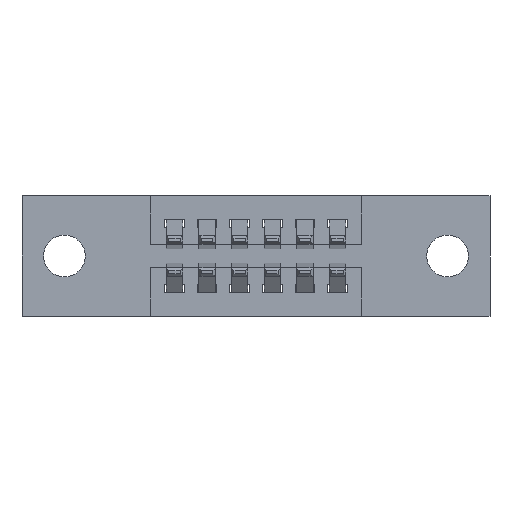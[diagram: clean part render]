
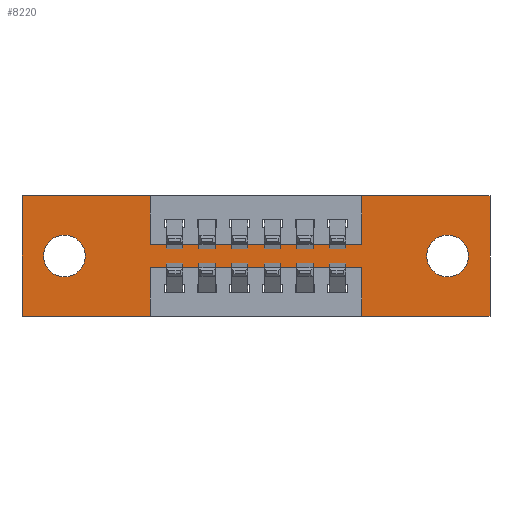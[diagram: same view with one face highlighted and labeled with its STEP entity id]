
A CAD part, front view. The second image highlights one B-rep face of the part: STEP entity #8220.
In plain terms, the highlighted planar face has unit normal (0, -1, 0).
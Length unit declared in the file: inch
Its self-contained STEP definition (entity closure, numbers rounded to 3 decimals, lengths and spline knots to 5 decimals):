
#97 = VERTEX_POINT ( 'NONE', #9076 ) ;
#116 = CARTESIAN_POINT ( 'NONE',  ( 1.305, 0., -0.249 ) ) ;
#131 = EDGE_CURVE ( 'NONE', #3369, #7412, #6602, .T. ) ;
#133 = LINE ( 'NONE', #6374, #9207 ) ;
#160 = CARTESIAN_POINT ( 'NONE',  ( 0.3925, 0., -0.22 ) ) ;
#163 = ORIENTED_EDGE ( 'NONE', *, *, #3945, .T. ) ;
#171 = DIRECTION ( 'NONE',  ( 0., 1., 0. ) ) ;
#182 = CARTESIAN_POINT ( 'NONE',  ( 0.3925, 0., -0.22 ) ) ;
#238 = CARTESIAN_POINT ( 'NONE',  ( 1.0425, 0., 0. ) ) ;
#259 = VECTOR ( 'NONE', #5340, 39.37008 ) ;
#364 = ORIENTED_EDGE ( 'NONE', *, *, #7373, .F. ) ;
#404 = DIRECTION ( 'NONE',  ( 0., 0., 1. ) ) ;
#483 = CARTESIAN_POINT ( 'NONE',  ( 0., 0., 0. ) ) ;
#496 = VERTEX_POINT ( 'NONE', #1741 ) ;
#575 = CARTESIAN_POINT ( 'NONE',  ( 1.305, 0., -0.185 ) ) ;
#585 = CARTESIAN_POINT ( 'NONE',  ( 0., 0., -0.37 ) ) ;
#763 = VECTOR ( 'NONE', #7663, 39.37008 ) ;
#859 = CIRCLE ( 'NONE', #6962, 0.064 ) ;
#992 = VERTEX_POINT ( 'NONE', #6722 ) ;
#1014 = VERTEX_POINT ( 'NONE', #182 ) ;
#1096 = CARTESIAN_POINT ( 'NONE',  ( 1.435, 0., 0. ) ) ;
#1185 = CARTESIAN_POINT ( 'NONE',  ( 1.0425, 0., -0.37 ) ) ;
#1200 = VERTEX_POINT ( 'NONE', #9214 ) ;
#1331 = VERTEX_POINT ( 'NONE', #1185 ) ;
#1410 = LINE ( 'NONE', #160, #9097 ) ;
#1441 = CARTESIAN_POINT ( 'NONE',  ( 0., 0., 0. ) ) ;
#1536 = CARTESIAN_POINT ( 'NONE',  ( 1.0425, 0., 0. ) ) ;
#1552 = EDGE_CURVE ( 'NONE', #97, #4890, #8085, .T. ) ;
#1741 = CARTESIAN_POINT ( 'NONE',  ( 1.0425, 0., -0.22 ) ) ;
#1841 = EDGE_LOOP ( 'NONE', ( #163, #6356 ) ) ;
#1906 = DIRECTION ( 'NONE',  ( 0., 0., -1. ) ) ;
#1920 = ORIENTED_EDGE ( 'NONE', *, *, #7056, .F. ) ;
#2049 = ORIENTED_EDGE ( 'NONE', *, *, #8981, .F. ) ;
#2123 = ORIENTED_EDGE ( 'NONE', *, *, #3942, .F. ) ;
#2144 = EDGE_CURVE ( 'NONE', #4339, #3369, #4245, .T. ) ;
#2242 = LINE ( 'NONE', #4698, #3986 ) ;
#2432 = EDGE_CURVE ( 'NONE', #7024, #2604, #133, .T. ) ;
#2460 = ORIENTED_EDGE ( 'NONE', *, *, #131, .F. ) ;
#2490 = EDGE_LOOP ( 'NONE', ( #2498, #3957, #364, #5927, #2123, #2460, #6778, #5373, #7607, #2049, #6780, #1920 ) ) ;
#2498 = ORIENTED_EDGE ( 'NONE', *, *, #2923, .F. ) ;
#2604 = VERTEX_POINT ( 'NONE', #5002 ) ;
#2683 = ORIENTED_EDGE ( 'NONE', *, *, #6058, .T. ) ;
#2715 = FACE_BOUND ( 'NONE', #1841, .T. ) ;
#2771 = EDGE_CURVE ( 'NONE', #496, #1014, #1410, .T. ) ;
#2819 = VECTOR ( 'NONE', #7422, 39.37008 ) ;
#2849 = LINE ( 'NONE', #1096, #4599 ) ;
#2923 = EDGE_CURVE ( 'NONE', #1014, #5334, #2242, .T. ) ;
#2934 = DIRECTION ( 'NONE',  ( 0., 1., 0. ) ) ;
#2957 = CIRCLE ( 'NONE', #9351, 0.064 ) ;
#3071 = EDGE_CURVE ( 'NONE', #992, #1331, #8165, .T. ) ;
#3369 = VERTEX_POINT ( 'NONE', #238 ) ;
#3648 = DIRECTION ( 'NONE',  ( 1., 0., 0. ) ) ;
#3942 = EDGE_CURVE ( 'NONE', #7412, #992, #2849, .T. ) ;
#3945 = EDGE_CURVE ( 'NONE', #8912, #9149, #2957, .T. ) ;
#3957 = ORIENTED_EDGE ( 'NONE', *, *, #2771, .F. ) ;
#3986 = VECTOR ( 'NONE', #5474, 39.37008 ) ;
#4027 = EDGE_LOOP ( 'NONE', ( #6821, #2683 ) ) ;
#4134 = PLANE ( 'NONE',  #7288 ) ;
#4175 = VERTEX_POINT ( 'NONE', #116 ) ;
#4245 = LINE ( 'NONE', #1536, #259 ) ;
#4307 = DIRECTION ( 'NONE',  ( -1., 0., 0. ) ) ;
#4339 = VERTEX_POINT ( 'NONE', #5133 ) ;
#4340 = AXIS2_PLACEMENT_3D ( 'NONE', #575, #2934, #7323 ) ;
#4599 = VECTOR ( 'NONE', #5661, 39.37008 ) ;
#4657 = DIRECTION ( 'NONE',  ( 0., 0., -1. ) ) ;
#4698 = CARTESIAN_POINT ( 'NONE',  ( 0.3925, 0., -0.37 ) ) ;
#4736 = CARTESIAN_POINT ( 'NONE',  ( 0., 0., 0. ) ) ;
#4763 = DIRECTION ( 'NONE',  ( 0., 0., 1. ) ) ;
#4890 = VERTEX_POINT ( 'NONE', #483 ) ;
#4946 = VECTOR ( 'NONE', #4959, 39.37008 ) ;
#4959 = DIRECTION ( 'NONE',  ( -1., 0., 0. ) ) ;
#5002 = CARTESIAN_POINT ( 'NONE',  ( 0.3925, 0., -0.15 ) ) ;
#5133 = CARTESIAN_POINT ( 'NONE',  ( 1.0425, 0., -0.15 ) ) ;
#5173 = LINE ( 'NONE', #585, #4946 ) ;
#5334 = VERTEX_POINT ( 'NONE', #8488 ) ;
#5340 = DIRECTION ( 'NONE',  ( 0., 0., 1. ) ) ;
#5373 = ORIENTED_EDGE ( 'NONE', *, *, #9313, .F. ) ;
#5474 = DIRECTION ( 'NONE',  ( 0., 0., -1. ) ) ;
#5500 = CARTESIAN_POINT ( 'NONE',  ( 1.0425, 0., -0.37 ) ) ;
#5510 = CARTESIAN_POINT ( 'NONE',  ( 0.3925, 0., 0. ) ) ;
#5661 = DIRECTION ( 'NONE',  ( 0., 0., -1. ) ) ;
#5853 = EDGE_CURVE ( 'NONE', #1200, #4175, #9607, .T. ) ;
#5877 = CARTESIAN_POINT ( 'NONE',  ( 0.3925, 0., -0.15 ) ) ;
#5927 = ORIENTED_EDGE ( 'NONE', *, *, #3071, .F. ) ;
#5988 = CARTESIAN_POINT ( 'NONE',  ( 0., 0., 0. ) ) ;
#6058 = EDGE_CURVE ( 'NONE', #4175, #1200, #9487, .T. ) ;
#6159 = CARTESIAN_POINT ( 'NONE',  ( 0.13, 0., -0.185 ) ) ;
#6207 = CARTESIAN_POINT ( 'NONE',  ( 1.305, 0., -0.185 ) ) ;
#6356 = ORIENTED_EDGE ( 'NONE', *, *, #6472, .T. ) ;
#6374 = CARTESIAN_POINT ( 'NONE',  ( 0.3925, 0., 0. ) ) ;
#6472 = EDGE_CURVE ( 'NONE', #9149, #8912, #859, .T. ) ;
#6602 = LINE ( 'NONE', #4736, #763 ) ;
#6722 = CARTESIAN_POINT ( 'NONE',  ( 1.435, 0., -0.37 ) ) ;
#6772 = DIRECTION ( 'NONE',  ( 0., 0., 1. ) ) ;
#6777 = LINE ( 'NONE', #5988, #2819 ) ;
#6778 = ORIENTED_EDGE ( 'NONE', *, *, #2144, .F. ) ;
#6780 = ORIENTED_EDGE ( 'NONE', *, *, #1552, .F. ) ;
#6789 = DIRECTION ( 'NONE',  ( -1., 0., 0. ) ) ;
#6821 = ORIENTED_EDGE ( 'NONE', *, *, #5853, .T. ) ;
#6891 = DIRECTION ( 'NONE',  ( 0., 0., 1. ) ) ;
#6917 = CARTESIAN_POINT ( 'NONE',  ( 0.13, 0., -0.185 ) ) ;
#6962 = AXIS2_PLACEMENT_3D ( 'NONE', #6917, #9078, #6891 ) ;
#6996 = VECTOR ( 'NONE', #3648, 39.37008 ) ;
#6999 = CARTESIAN_POINT ( 'NONE',  ( 1.435, 0., 0. ) ) ;
#7024 = VERTEX_POINT ( 'NONE', #5510 ) ;
#7056 = EDGE_CURVE ( 'NONE', #5334, #97, #5173, .T. ) ;
#7288 = AXIS2_PLACEMENT_3D ( 'NONE', #9410, #7326, #8675 ) ;
#7323 = DIRECTION ( 'NONE',  ( 0., 0., -1. ) ) ;
#7326 = DIRECTION ( 'NONE',  ( 0., -1., 0. ) ) ;
#7373 = EDGE_CURVE ( 'NONE', #1331, #496, #7840, .T. ) ;
#7412 = VERTEX_POINT ( 'NONE', #6999 ) ;
#7422 = DIRECTION ( 'NONE',  ( 1., 0., 0. ) ) ;
#7458 = AXIS2_PLACEMENT_3D ( 'NONE', #6207, #171, #4657 ) ;
#7607 = ORIENTED_EDGE ( 'NONE', *, *, #2432, .F. ) ;
#7663 = DIRECTION ( 'NONE',  ( 1., 0., 0. ) ) ;
#7840 = LINE ( 'NONE', #5500, #8644 ) ;
#8000 = CARTESIAN_POINT ( 'NONE',  ( 0., 0., -0.37 ) ) ;
#8014 = CARTESIAN_POINT ( 'NONE',  ( 0.13, 0., -0.121 ) ) ;
#8035 = LINE ( 'NONE', #5877, #6996 ) ;
#8085 = LINE ( 'NONE', #1441, #9583 ) ;
#8165 = LINE ( 'NONE', #8000, #9089 ) ;
#8170 = FACE_OUTER_BOUND ( 'NONE', #2490, .T. ) ;
#8220 = ADVANCED_FACE ( 'NONE', ( #9551, #2715, #8170 ), #4134, .T. ) ;
#8488 = CARTESIAN_POINT ( 'NONE',  ( 0.3925, 0., -0.37 ) ) ;
#8582 = CARTESIAN_POINT ( 'NONE',  ( 0.13, 0., -0.249 ) ) ;
#8644 = VECTOR ( 'NONE', #4763, 39.37008 ) ;
#8675 = DIRECTION ( 'NONE',  ( 0., 0., -1. ) ) ;
#8912 = VERTEX_POINT ( 'NONE', #8014 ) ;
#8981 = EDGE_CURVE ( 'NONE', #4890, #7024, #6777, .T. ) ;
#9076 = CARTESIAN_POINT ( 'NONE',  ( 0., 0., -0.37 ) ) ;
#9078 = DIRECTION ( 'NONE',  ( 0., 1., 0. ) ) ;
#9089 = VECTOR ( 'NONE', #4307, 39.37008 ) ;
#9097 = VECTOR ( 'NONE', #6789, 39.37008 ) ;
#9149 = VERTEX_POINT ( 'NONE', #8582 ) ;
#9207 = VECTOR ( 'NONE', #1906, 39.37008 ) ;
#9214 = CARTESIAN_POINT ( 'NONE',  ( 1.305, 0., -0.121 ) ) ;
#9313 = EDGE_CURVE ( 'NONE', #2604, #4339, #8035, .T. ) ;
#9317 = DIRECTION ( 'NONE',  ( 0., 1., 0. ) ) ;
#9351 = AXIS2_PLACEMENT_3D ( 'NONE', #6159, #9317, #404 ) ;
#9410 = CARTESIAN_POINT ( 'NONE',  ( 0., 0., -0.37 ) ) ;
#9487 = CIRCLE ( 'NONE', #7458, 0.064 ) ;
#9551 = FACE_BOUND ( 'NONE', #4027, .T. ) ;
#9583 = VECTOR ( 'NONE', #6772, 39.37008 ) ;
#9607 = CIRCLE ( 'NONE', #4340, 0.064 ) ;
